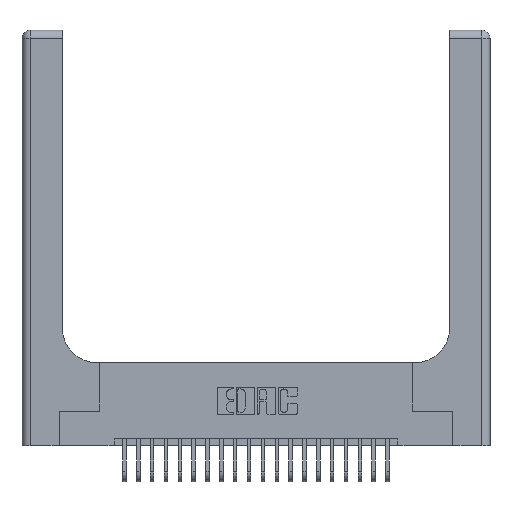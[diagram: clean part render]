
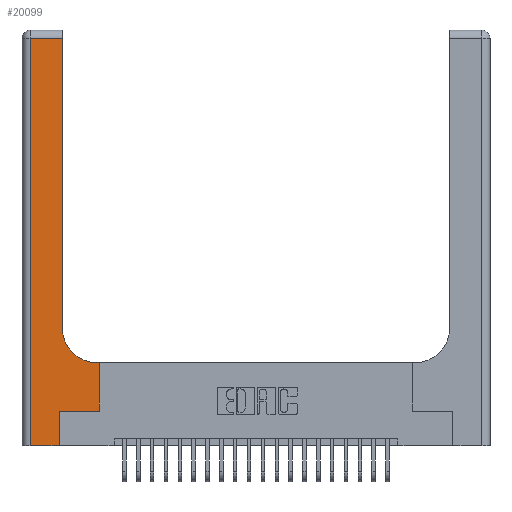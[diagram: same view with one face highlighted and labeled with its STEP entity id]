
A CAD part, top view. The second image highlights one B-rep face of the part: STEP entity #20099.
In plain terms, the highlighted planar face has unit normal (0, 0, 1).
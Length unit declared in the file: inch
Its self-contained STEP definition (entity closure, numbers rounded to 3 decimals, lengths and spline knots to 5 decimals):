
#167 = VECTOR ( 'NONE', #14276, 39.37008 ) ;
#253 = EDGE_CURVE ( 'NONE', #19966, #17565, #11119, .T. ) ;
#409 = CARTESIAN_POINT ( 'NONE',  ( 0.5415, 0.85, 0.37 ) ) ;
#1276 = LINE ( 'NONE', #3961, #23777 ) ;
#1445 = LINE ( 'NONE', #23737, #3956 ) ;
#1874 = LINE ( 'NONE', #7910, #8956 ) ;
#2141 = CARTESIAN_POINT ( 'NONE',  ( 0., 3., 0.37 ) ) ;
#2215 = EDGE_CURVE ( 'NONE', #17565, #10655, #1445, .T. ) ;
#2256 = DIRECTION ( 'NONE',  ( 1., 0., 0. ) ) ;
#3535 = ORIENTED_EDGE ( 'NONE', *, *, #25327, .T. ) ;
#3726 = ORIENTED_EDGE ( 'NONE', *, *, #2215, .T. ) ;
#3888 = PLANE ( 'NONE',  #10695 ) ;
#3956 = VECTOR ( 'NONE', #25467, 39.37008 ) ;
#3961 = CARTESIAN_POINT ( 'NONE',  ( 0.06, 3., 0.37 ) ) ;
#4143 = EDGE_CURVE ( 'NONE', #10517, #13068, #11269, .T. ) ;
#5919 = AXIS2_PLACEMENT_3D ( 'NONE', #409, #6319, #2256 ) ;
#6319 = DIRECTION ( 'NONE',  ( 0., 0., -1. ) ) ;
#6939 = CARTESIAN_POINT ( 'NONE',  ( 0., 0., 0.37 ) ) ;
#7170 = CARTESIAN_POINT ( 'NONE',  ( 0.269, 0., 0.37 ) ) ;
#7334 = VECTOR ( 'NONE', #17007, 39.37008 ) ;
#7661 = LINE ( 'NONE', #20782, #7334 ) ;
#7901 = DIRECTION ( 'NONE',  ( 0., -1., 0. ) ) ;
#7910 = CARTESIAN_POINT ( 'NONE',  ( 0.5585, 0.25, 0.37 ) ) ;
#8165 = ORIENTED_EDGE ( 'NONE', *, *, #253, .T. ) ;
#8860 = EDGE_CURVE ( 'NONE', #14122, #10517, #10529, .T. ) ;
#8956 = VECTOR ( 'NONE', #19868, 39.37008 ) ;
#9222 = DIRECTION ( 'NONE',  ( 0., 1., 0. ) ) ;
#9266 = CARTESIAN_POINT ( 'NONE',  ( 0.2915, 0.6, 0.37 ) ) ;
#9414 = EDGE_CURVE ( 'NONE', #11040, #16020, #1276, .T. ) ;
#10219 = CARTESIAN_POINT ( 'NONE',  ( 0.269, 0.25, 0.37 ) ) ;
#10517 = VERTEX_POINT ( 'NONE', #15793 ) ;
#10529 = LINE ( 'NONE', #9266, #20117 ) ;
#10550 = ORIENTED_EDGE ( 'NONE', *, *, #8860, .T. ) ;
#10655 = VERTEX_POINT ( 'NONE', #19906 ) ;
#10695 = AXIS2_PLACEMENT_3D ( 'NONE', #2141, #23491, #21596 ) ;
#11040 = VERTEX_POINT ( 'NONE', #20939 ) ;
#11119 = LINE ( 'NONE', #7170, #16051 ) ;
#11269 = CIRCLE ( 'NONE', #5919, 0.25 ) ;
#11652 = VECTOR ( 'NONE', #22736, 39.37008 ) ;
#11706 = EDGE_CURVE ( 'NONE', #16020, #19966, #16897, .T. ) ;
#12192 = LINE ( 'NONE', #14196, #167 ) ;
#13068 = VERTEX_POINT ( 'NONE', #17229 ) ;
#14122 = VERTEX_POINT ( 'NONE', #25291 ) ;
#14196 = CARTESIAN_POINT ( 'NONE',  ( 0.2915, 3., 0.37 ) ) ;
#14276 = DIRECTION ( 'NONE',  ( 0., 1., 0. ) ) ;
#15111 = VERTEX_POINT ( 'NONE', #21756 ) ;
#15428 = ORIENTED_EDGE ( 'NONE', *, *, #9414, .T. ) ;
#15793 = CARTESIAN_POINT ( 'NONE',  ( 0.5415, 0.6, 0.37 ) ) ;
#16020 = VERTEX_POINT ( 'NONE', #22562 ) ;
#16051 = VECTOR ( 'NONE', #9222, 39.37008 ) ;
#16897 = LINE ( 'NONE', #6939, #11652 ) ;
#17007 = DIRECTION ( 'NONE',  ( -1., 0., 0. ) ) ;
#17229 = CARTESIAN_POINT ( 'NONE',  ( 0.2915, 0.85, 0.37 ) ) ;
#17565 = VERTEX_POINT ( 'NONE', #10219 ) ;
#19266 = CARTESIAN_POINT ( 'NONE',  ( 0.269, 0., 0.37 ) ) ;
#19590 = EDGE_CURVE ( 'NONE', #13068, #15111, #12192, .T. ) ;
#19856 = ORIENTED_EDGE ( 'NONE', *, *, #23890, .T. ) ;
#19868 = DIRECTION ( 'NONE',  ( 0., 1., 0. ) ) ;
#19906 = CARTESIAN_POINT ( 'NONE',  ( 0.5585, 0.25, 0.37 ) ) ;
#19966 = VERTEX_POINT ( 'NONE', #19266 ) ;
#20099 = ADVANCED_FACE ( 'NONE', ( #22945 ), #3888, .F. ) ;
#20117 = VECTOR ( 'NONE', #22844, 39.37008 ) ;
#20782 = CARTESIAN_POINT ( 'NONE',  ( 0., 2.94, 0.37 ) ) ;
#20939 = CARTESIAN_POINT ( 'NONE',  ( 0.06, 2.94, 0.37 ) ) ;
#21144 = ORIENTED_EDGE ( 'NONE', *, *, #19590, .T. ) ;
#21596 = DIRECTION ( 'NONE',  ( -1., 0., 0. ) ) ;
#21673 = EDGE_LOOP ( 'NONE', ( #21144, #3535, #15428, #23170, #8165, #3726, #19856, #10550, #25490 ) ) ;
#21756 = CARTESIAN_POINT ( 'NONE',  ( 0.2915, 2.94, 0.37 ) ) ;
#22562 = CARTESIAN_POINT ( 'NONE',  ( 0.06, 0., 0.37 ) ) ;
#22736 = DIRECTION ( 'NONE',  ( 1., 0., 0. ) ) ;
#22844 = DIRECTION ( 'NONE',  ( -1., 0., 0. ) ) ;
#22945 = FACE_OUTER_BOUND ( 'NONE', #21673, .T. ) ;
#23170 = ORIENTED_EDGE ( 'NONE', *, *, #11706, .T. ) ;
#23491 = DIRECTION ( 'NONE',  ( 0., 0., -1. ) ) ;
#23737 = CARTESIAN_POINT ( 'NONE',  ( 0.269, 0.25, 0.37 ) ) ;
#23777 = VECTOR ( 'NONE', #7901, 39.37008 ) ;
#23890 = EDGE_CURVE ( 'NONE', #10655, #14122, #1874, .T. ) ;
#25291 = CARTESIAN_POINT ( 'NONE',  ( 0.5585, 0.6, 0.37 ) ) ;
#25327 = EDGE_CURVE ( 'NONE', #15111, #11040, #7661, .T. ) ;
#25467 = DIRECTION ( 'NONE',  ( 1., 0., 0. ) ) ;
#25490 = ORIENTED_EDGE ( 'NONE', *, *, #4143, .T. ) ;
